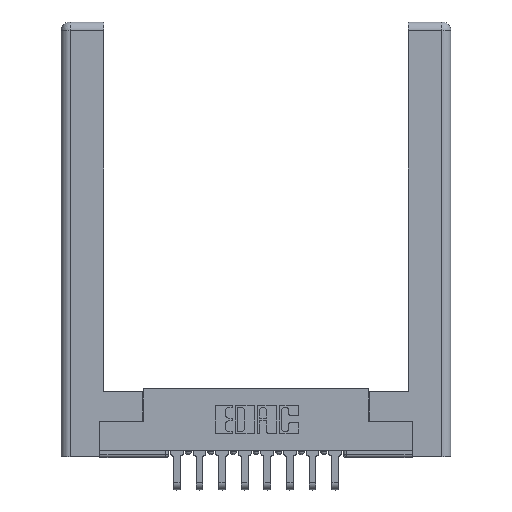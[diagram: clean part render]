
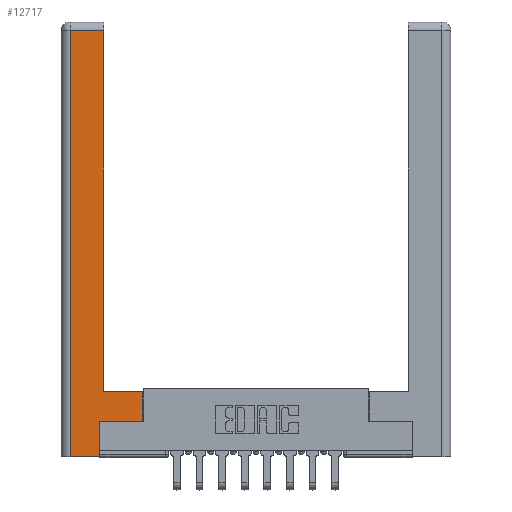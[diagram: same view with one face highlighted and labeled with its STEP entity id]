
A CAD part, top view. The second image highlights one B-rep face of the part: STEP entity #12717.
In plain terms, the highlighted planar face has unit normal (0, 0, 1).
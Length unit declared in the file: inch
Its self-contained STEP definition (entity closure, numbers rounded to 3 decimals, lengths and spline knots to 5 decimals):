
#399 = VERTEX_POINT ( 'NONE', #8393 ) ;
#460 = EDGE_CURVE ( 'NONE', #8519, #1886, #5211, .T. ) ;
#739 = PLANE ( 'NONE',  #13475 ) ;
#815 = LINE ( 'NONE', #5585, #15140 ) ;
#997 = VERTEX_POINT ( 'NONE', #10234 ) ;
#1241 = CARTESIAN_POINT ( 'NONE',  ( 0.295, 0.45, 0. ) ) ;
#1306 = LINE ( 'NONE', #9930, #12724 ) ;
#1412 = CARTESIAN_POINT ( 'NONE',  ( 0.265, 0., 0. ) ) ;
#1886 = VERTEX_POINT ( 'NONE', #8691 ) ;
#2216 = VERTEX_POINT ( 'NONE', #7066 ) ;
#2243 = CARTESIAN_POINT ( 'NONE',  ( 0.265, 0., 0. ) ) ;
#2599 = LINE ( 'NONE', #1412, #2703 ) ;
#2703 = VECTOR ( 'NONE', #5083, 39.37008 ) ;
#2712 = CARTESIAN_POINT ( 'NONE',  ( 0.0615, 2.94, 0. ) ) ;
#2883 = EDGE_CURVE ( 'NONE', #997, #2216, #15340, .T. ) ;
#3293 = FACE_OUTER_BOUND ( 'NONE', #5114, .T. ) ;
#3496 = DIRECTION ( 'NONE',  ( -1., 0., 0. ) ) ;
#4008 = DIRECTION ( 'NONE',  ( 0., 1., 0. ) ) ;
#4041 = ORIENTED_EDGE ( 'NONE', *, *, #11992, .T. ) ;
#4043 = CARTESIAN_POINT ( 'NONE',  ( 0.0615, 0., 0. ) ) ;
#4168 = LINE ( 'NONE', #5401, #8619 ) ;
#4551 = ORIENTED_EDGE ( 'NONE', *, *, #12949, .T. ) ;
#4622 = ORIENTED_EDGE ( 'NONE', *, *, #460, .T. ) ;
#4646 = LINE ( 'NONE', #9396, #14711 ) ;
#4894 = DIRECTION ( 'NONE',  ( 0., 1., 0. ) ) ;
#4975 = DIRECTION ( 'NONE',  ( 0., -1., 0. ) ) ;
#5083 = DIRECTION ( 'NONE',  ( 1., 0., 0. ) ) ;
#5114 = EDGE_LOOP ( 'NONE', ( #12137, #4041, #4622, #13651, #7439, #12165, #14177, #4551 ) ) ;
#5177 = EDGE_CURVE ( 'NONE', #2216, #10379, #4168, .T. ) ;
#5211 = LINE ( 'NONE', #4043, #11890 ) ;
#5401 = CARTESIAN_POINT ( 'NONE',  ( 0.565, 0.45, 0. ) ) ;
#5585 = CARTESIAN_POINT ( 'NONE',  ( 0.265, 0.245, 0. ) ) ;
#5850 = CARTESIAN_POINT ( 'NONE',  ( 0.295, 3., 0. ) ) ;
#6317 = VERTEX_POINT ( 'NONE', #2243 ) ;
#6834 = DIRECTION ( 'NONE',  ( 0., 1., 0. ) ) ;
#7066 = CARTESIAN_POINT ( 'NONE',  ( 0.565, 0.245, 0. ) ) ;
#7141 = CARTESIAN_POINT ( 'NONE',  ( 0.565, 0.45, 0. ) ) ;
#7439 = ORIENTED_EDGE ( 'NONE', *, *, #8744, .T. ) ;
#8215 = EDGE_CURVE ( 'NONE', #1886, #6317, #2599, .T. ) ;
#8381 = EDGE_CURVE ( 'NONE', #11058, #399, #9424, .T. ) ;
#8393 = CARTESIAN_POINT ( 'NONE',  ( 0.295, 2.94, 0. ) ) ;
#8519 = VERTEX_POINT ( 'NONE', #2712 ) ;
#8529 = DIRECTION ( 'NONE',  ( -1., 0., 0. ) ) ;
#8619 = VECTOR ( 'NONE', #4008, 39.37008 ) ;
#8660 = VECTOR ( 'NONE', #4894, 39.37008 ) ;
#8691 = CARTESIAN_POINT ( 'NONE',  ( 0.0615, 0., 0. ) ) ;
#8744 = EDGE_CURVE ( 'NONE', #6317, #997, #815, .T. ) ;
#9396 = CARTESIAN_POINT ( 'NONE',  ( 0.0615, 2.94, 0. ) ) ;
#9424 = LINE ( 'NONE', #5850, #8660 ) ;
#9930 = CARTESIAN_POINT ( 'NONE',  ( 0.295, 0.45, 0. ) ) ;
#10220 = VECTOR ( 'NONE', #10596, 39.37008 ) ;
#10234 = CARTESIAN_POINT ( 'NONE',  ( 0.265, 0.245, 0. ) ) ;
#10379 = VERTEX_POINT ( 'NONE', #7141 ) ;
#10596 = DIRECTION ( 'NONE',  ( 1., 0., 0. ) ) ;
#11058 = VERTEX_POINT ( 'NONE', #1241 ) ;
#11500 = DIRECTION ( 'NONE',  ( 0., 0., -1. ) ) ;
#11688 = CARTESIAN_POINT ( 'NONE',  ( 0.565, 0.245, 0. ) ) ;
#11890 = VECTOR ( 'NONE', #4975, 39.37008 ) ;
#11992 = EDGE_CURVE ( 'NONE', #399, #8519, #4646, .T. ) ;
#12137 = ORIENTED_EDGE ( 'NONE', *, *, #8381, .T. ) ;
#12165 = ORIENTED_EDGE ( 'NONE', *, *, #2883, .T. ) ;
#12717 = ADVANCED_FACE ( 'NONE', ( #3293 ), #739, .F. ) ;
#12724 = VECTOR ( 'NONE', #8529, 39.37008 ) ;
#12949 = EDGE_CURVE ( 'NONE', #10379, #11058, #1306, .T. ) ;
#13475 = AXIS2_PLACEMENT_3D ( 'NONE', #13675, #11500, #14915 ) ;
#13651 = ORIENTED_EDGE ( 'NONE', *, *, #8215, .T. ) ;
#13675 = CARTESIAN_POINT ( 'NONE',  ( 0., 0., 0. ) ) ;
#14177 = ORIENTED_EDGE ( 'NONE', *, *, #5177, .T. ) ;
#14711 = VECTOR ( 'NONE', #3496, 39.37008 ) ;
#14915 = DIRECTION ( 'NONE',  ( -1., 0., 0. ) ) ;
#15140 = VECTOR ( 'NONE', #6834, 39.37008 ) ;
#15340 = LINE ( 'NONE', #11688, #10220 ) ;
